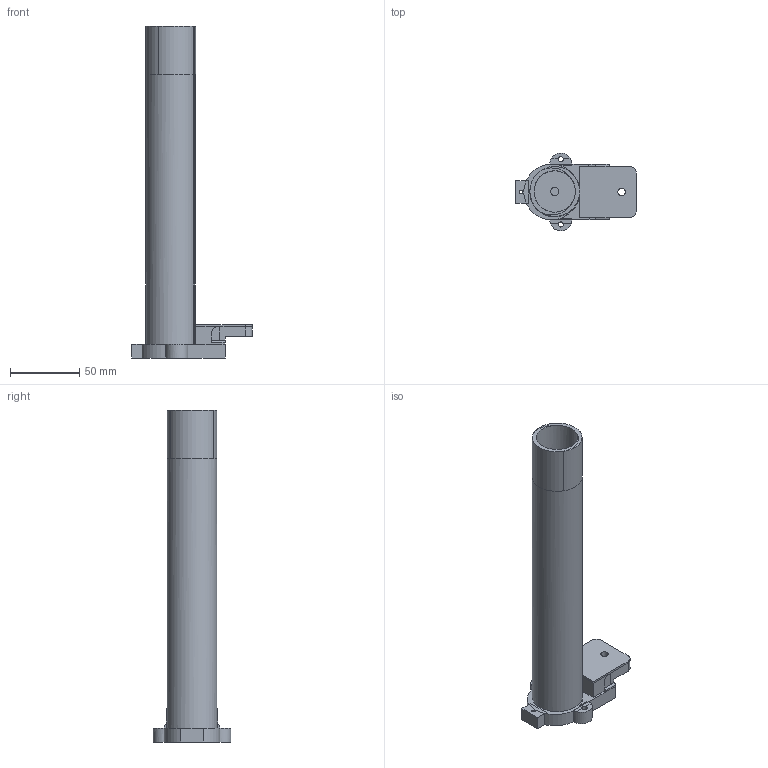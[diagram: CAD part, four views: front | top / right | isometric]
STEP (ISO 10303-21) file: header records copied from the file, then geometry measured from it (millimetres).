
FILE_DESCRIPTION(('FreeCAD Model'),'2;1');
FILE_NAME('ap9 buffer tube abs,peek,polymide,nylon no support.step','2018-08-08T20:33:21',('Author' ),(''),'Open CASCADE STEP processor 6.8','FreeCAD','Unknown');
FILE_SCHEMA(('AUTOMOTIVE_DESIGN_CC2 { 1 2 10303 214 -1 1 5 4 }'));
Length unit declared in the file: millimetre
Products named in the file (1): Chamfer
Bounding box: 86.94 x 56.2 x 240 mm (x, y, z)
Volume: 158321.9 mm3; surface area: 55334.3 mm2
Topology: 1 solids, 1 shells, 102 faces, 250 edges, 153 vertices
Faces by surface type: plane 69, cylinder 32, bspline 1
Full cylindrical faces by diameter (mm): 2.4 x1, 3.7 x2, 5.5 x3, 17.93 x1, 26 x1, 30 x2
Entity records: 6558 total; most frequent: CARTESIAN_POINT 1668, DIRECTION 907, ORIENTED_EDGE 500, PCURVE 500, DEFINITIONAL_REPRESENTATION 500, LINE 465, VECTOR 465, EDGE_CURVE 250
